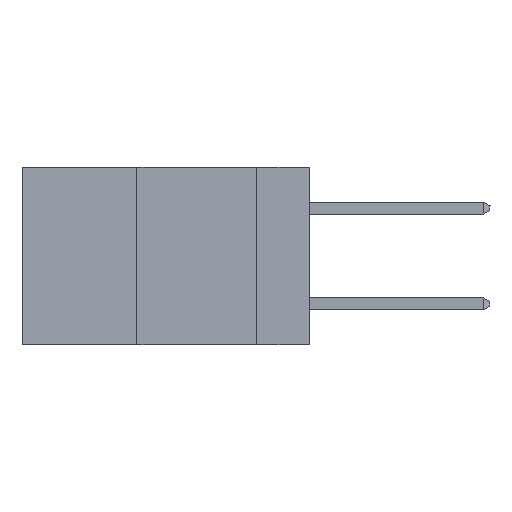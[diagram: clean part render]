
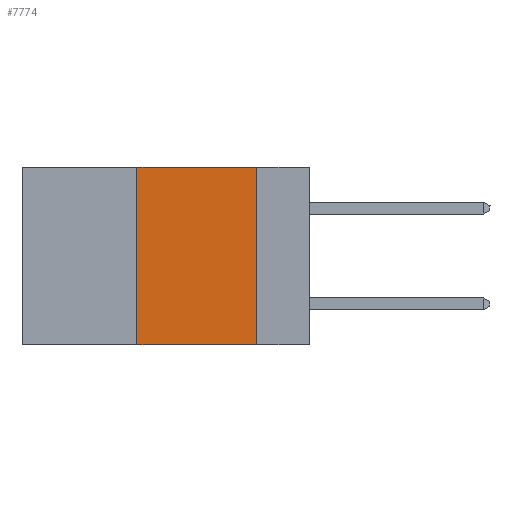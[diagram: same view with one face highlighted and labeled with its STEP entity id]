
A CAD part, left-side view. The second image highlights one B-rep face of the part: STEP entity #7774.
In plain terms, the highlighted planar face has unit normal (-1, 0, 0).
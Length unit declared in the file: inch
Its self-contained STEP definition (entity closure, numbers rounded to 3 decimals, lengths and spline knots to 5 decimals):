
#48 = CARTESIAN_POINT ( 'NONE',  ( 0., 0.6, 0. ) ) ;
#475 = CARTESIAN_POINT ( 'NONE',  ( 0., 0.36, 0. ) ) ;
#643 = LINE ( 'NONE', #10800, #26593 ) ;
#914 = EDGE_LOOP ( 'NONE', ( #15886, #21332, #26039, #14511 ) ) ;
#2762 = CARTESIAN_POINT ( 'NONE',  ( 0., 0.11, 0. ) ) ;
#3232 = FACE_OUTER_BOUND ( 'NONE', #914, .T. ) ;
#4885 = LINE ( 'NONE', #30362, #30744 ) ;
#5212 = LINE ( 'NONE', #48, #30440 ) ;
#5580 = PLANE ( 'NONE',  #27253 ) ;
#7774 = ADVANCED_FACE ( 'NONE', ( #3232 ), #5580, .F. ) ;
#8399 = CARTESIAN_POINT ( 'NONE',  ( 0., 0.6, 0. ) ) ;
#8719 = DIRECTION ( 'NONE',  ( 1., 0., 0. ) ) ;
#9532 = EDGE_CURVE ( 'NONE', #26778, #14941, #5212, .T. ) ;
#9737 = CARTESIAN_POINT ( 'NONE',  ( 0., 0.36, 0. ) ) ;
#10465 = LINE ( 'NONE', #475, #28412 ) ;
#10800 = CARTESIAN_POINT ( 'NONE',  ( 0., 0.11, 0. ) ) ;
#12813 = DIRECTION ( 'NONE',  ( 0., 0., -1. ) ) ;
#13895 = VERTEX_POINT ( 'NONE', #22547 ) ;
#14511 = ORIENTED_EDGE ( 'NONE', *, *, #17874, .T. ) ;
#14941 = VERTEX_POINT ( 'NONE', #2762 ) ;
#15886 = ORIENTED_EDGE ( 'NONE', *, *, #22132, .F. ) ;
#17874 = EDGE_CURVE ( 'NONE', #21708, #13895, #4885, .T. ) ;
#21332 = ORIENTED_EDGE ( 'NONE', *, *, #9532, .F. ) ;
#21708 = VERTEX_POINT ( 'NONE', #26146 ) ;
#22132 = EDGE_CURVE ( 'NONE', #14941, #13895, #643, .T. ) ;
#22547 = CARTESIAN_POINT ( 'NONE',  ( 0., 0.11, -0.37 ) ) ;
#22697 = DIRECTION ( 'NONE',  ( 0., -1., 0. ) ) ;
#23607 = DIRECTION ( 'NONE',  ( 0., 0., 1. ) ) ;
#26039 = ORIENTED_EDGE ( 'NONE', *, *, #26057, .F. ) ;
#26057 = EDGE_CURVE ( 'NONE', #21708, #26778, #10465, .T. ) ;
#26146 = CARTESIAN_POINT ( 'NONE',  ( 0., 0.36, -0.37 ) ) ;
#26363 = DIRECTION ( 'NONE',  ( 0., 0., -1. ) ) ;
#26593 = VECTOR ( 'NONE', #12813, 39.37008 ) ;
#26778 = VERTEX_POINT ( 'NONE', #9737 ) ;
#27253 = AXIS2_PLACEMENT_3D ( 'NONE', #8399, #8719, #26363 ) ;
#27529 = DIRECTION ( 'NONE',  ( 0., -1., 0. ) ) ;
#28412 = VECTOR ( 'NONE', #23607, 39.37008 ) ;
#30362 = CARTESIAN_POINT ( 'NONE',  ( 0., 0.6, -0.37 ) ) ;
#30440 = VECTOR ( 'NONE', #22697, 39.37008 ) ;
#30744 = VECTOR ( 'NONE', #27529, 39.37008 ) ;
